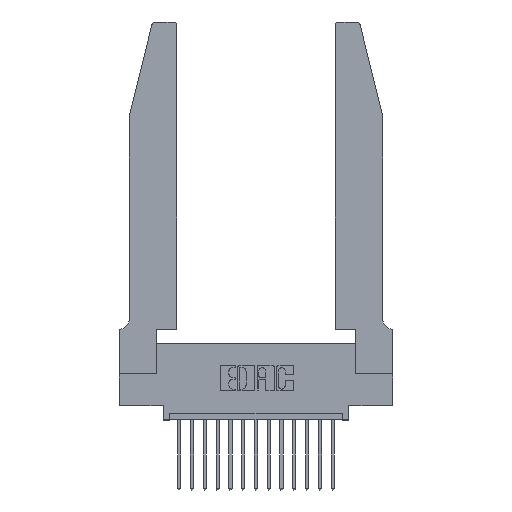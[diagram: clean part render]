
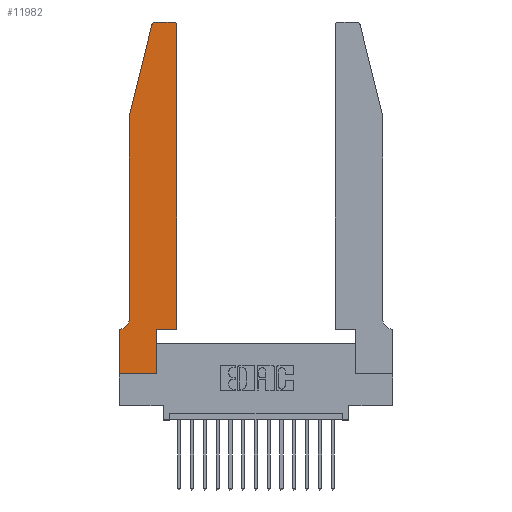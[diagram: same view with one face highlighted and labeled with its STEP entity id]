
A CAD part, top view. The second image highlights one B-rep face of the part: STEP entity #11982.
In plain terms, the highlighted planar face has unit normal (0, 0, 1).
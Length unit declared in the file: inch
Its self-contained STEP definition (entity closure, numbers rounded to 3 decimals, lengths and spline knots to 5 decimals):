
#133 = AXIS2_PLACEMENT_3D ( 'NONE', #11825, #15166, #6488 ) ;
#230 = EDGE_CURVE ( 'NONE', #1227, #12452, #915, .T. ) ;
#235 = CARTESIAN_POINT ( 'NONE',  ( 0., 0., 0.37 ) ) ;
#399 = CARTESIAN_POINT ( 'NONE',  ( 0.4505, 0.35, 0.37 ) ) ;
#492 = VERTEX_POINT ( 'NONE', #2204 ) ;
#555 = DIRECTION ( 'NONE',  ( -1., 0., 0. ) ) ;
#572 = CIRCLE ( 'NONE', #10017, 0.03 ) ;
#741 = LINE ( 'NONE', #235, #9506 ) ;
#759 = EDGE_CURVE ( 'NONE', #11024, #836, #6072, .T. ) ;
#790 = LINE ( 'NONE', #4311, #17644 ) ;
#828 = CARTESIAN_POINT ( 'NONE',  ( 0.0755, 2., 0.37 ) ) ;
#836 = VERTEX_POINT ( 'NONE', #18049 ) ;
#915 = LINE ( 'NONE', #828, #8326 ) ;
#1227 = VERTEX_POINT ( 'NONE', #9292 ) ;
#1251 = DIRECTION ( 'NONE',  ( 0., -1., 0. ) ) ;
#1268 = CIRCLE ( 'NONE', #8624, 0.07 ) ;
#1485 = EDGE_CURVE ( 'NONE', #11326, #2043, #12136, .T. ) ;
#1610 = ORIENTED_EDGE ( 'NONE', *, *, #5143, .T. ) ;
#1847 = CARTESIAN_POINT ( 'NONE',  ( 0.0755, 0.35, 0.37 ) ) ;
#1971 = EDGE_CURVE ( 'NONE', #2043, #492, #11453, .T. ) ;
#2043 = VERTEX_POINT ( 'NONE', #17514 ) ;
#2071 = ORIENTED_EDGE ( 'NONE', *, *, #759, .T. ) ;
#2204 = CARTESIAN_POINT ( 'NONE',  ( 0.4505, 0.35, 0.37 ) ) ;
#2301 = AXIS2_PLACEMENT_3D ( 'NONE', #8332, #8388, #2552 ) ;
#2552 = DIRECTION ( 'NONE',  ( 1., 0., 0. ) ) ;
#2676 = VECTOR ( 'NONE', #11862, 39.37008 ) ;
#3142 = CARTESIAN_POINT ( 'NONE',  ( 0.0755, 0.42, 0.37 ) ) ;
#3165 = DIRECTION ( 'NONE',  ( -1., 0., 0. ) ) ;
#3204 = CARTESIAN_POINT ( 'NONE',  ( 0., 0., 0.37 ) ) ;
#3379 = ORIENTED_EDGE ( 'NONE', *, *, #9868, .T. ) ;
#3469 = ORIENTED_EDGE ( 'NONE', *, *, #7093, .T. ) ;
#3857 = ORIENTED_EDGE ( 'NONE', *, *, #1971, .T. ) ;
#4170 = LINE ( 'NONE', #399, #8900 ) ;
#4178 = EDGE_CURVE ( 'NONE', #12461, #1227, #572, .T. ) ;
#4311 = CARTESIAN_POINT ( 'NONE',  ( 0.0755, 2., 0.37 ) ) ;
#4989 = DIRECTION ( 'NONE',  ( 0., 1., 0. ) ) ;
#5143 = EDGE_CURVE ( 'NONE', #12452, #11665, #790, .T. ) ;
#5204 = EDGE_CURVE ( 'NONE', #12669, #11326, #18302, .T. ) ;
#5235 = FACE_OUTER_BOUND ( 'NONE', #9716, .T. ) ;
#5941 = CARTESIAN_POINT ( 'NONE',  ( 0., 0., 0.37 ) ) ;
#6072 = CIRCLE ( 'NONE', #133, 0.03 ) ;
#6348 = ORIENTED_EDGE ( 'NONE', *, *, #230, .T. ) ;
#6377 = CARTESIAN_POINT ( 'NONE',  ( 0.0055, 0.35, 0.37 ) ) ;
#6461 = DIRECTION ( 'NONE',  ( -0.239, -0.971, 0. ) ) ;
#6488 = DIRECTION ( 'NONE',  ( 1., 0., 0. ) ) ;
#6499 = CARTESIAN_POINT ( 'NONE',  ( 0.284, 2.72, 0.37 ) ) ;
#6791 = CARTESIAN_POINT ( 'NONE',  ( 0.284, 2.75, 0.37 ) ) ;
#6950 = PLANE ( 'NONE',  #2301 ) ;
#7093 = EDGE_CURVE ( 'NONE', #492, #11024, #4170, .T. ) ;
#7434 = DIRECTION ( 'NONE',  ( 0., -1., 0. ) ) ;
#8117 = VERTEX_POINT ( 'NONE', #6377 ) ;
#8326 = VECTOR ( 'NONE', #6461, 39.37008 ) ;
#8332 = CARTESIAN_POINT ( 'NONE',  ( 0., 0.35, 0.37 ) ) ;
#8388 = DIRECTION ( 'NONE',  ( 0., 0., 1. ) ) ;
#8523 = VECTOR ( 'NONE', #4989, 39.37008 ) ;
#8624 = AXIS2_PLACEMENT_3D ( 'NONE', #13584, #9450, #16480 ) ;
#8760 = ORIENTED_EDGE ( 'NONE', *, *, #9781, .T. ) ;
#8900 = VECTOR ( 'NONE', #10963, 39.37008 ) ;
#9292 = CARTESIAN_POINT ( 'NONE',  ( 0.25487, 2.72718, 0.37 ) ) ;
#9450 = DIRECTION ( 'NONE',  ( 0., 0., -1. ) ) ;
#9506 = VECTOR ( 'NONE', #7434, 39.37008 ) ;
#9716 = EDGE_LOOP ( 'NONE', ( #15993, #14338, #6348, #1610, #3379, #8760, #15944, #17517, #10723, #3857, #3469, #2071 ) ) ;
#9781 = EDGE_CURVE ( 'NONE', #8117, #17095, #9831, .T. ) ;
#9831 = LINE ( 'NONE', #1847, #15447 ) ;
#9868 = EDGE_CURVE ( 'NONE', #11665, #8117, #1268, .T. ) ;
#10017 = AXIS2_PLACEMENT_3D ( 'NONE', #6499, #18011, #17128 ) ;
#10723 = ORIENTED_EDGE ( 'NONE', *, *, #1485, .T. ) ;
#10909 = CARTESIAN_POINT ( 'NONE',  ( 0.2865, 0.35, 0.37 ) ) ;
#10963 = DIRECTION ( 'NONE',  ( 0., 1., 0. ) ) ;
#11024 = VERTEX_POINT ( 'NONE', #14594 ) ;
#11326 = VERTEX_POINT ( 'NONE', #13890 ) ;
#11453 = LINE ( 'NONE', #14544, #2676 ) ;
#11665 = VERTEX_POINT ( 'NONE', #3142 ) ;
#11825 = CARTESIAN_POINT ( 'NONE',  ( 0.4205, 2.72, 0.37 ) ) ;
#11862 = DIRECTION ( 'NONE',  ( 1., 0., 0. ) ) ;
#11982 = ADVANCED_FACE ( 'NONE', ( #5235 ), #6950, .T. ) ;
#12136 = LINE ( 'NONE', #10909, #8523 ) ;
#12452 = VERTEX_POINT ( 'NONE', #18240 ) ;
#12461 = VERTEX_POINT ( 'NONE', #6791 ) ;
#12669 = VERTEX_POINT ( 'NONE', #3204 ) ;
#12739 = EDGE_CURVE ( 'NONE', #836, #12461, #14475, .T. ) ;
#13584 = CARTESIAN_POINT ( 'NONE',  ( 0.0055, 0.42, 0.37 ) ) ;
#13890 = CARTESIAN_POINT ( 'NONE',  ( 0.2865, 0., 0.37 ) ) ;
#14338 = ORIENTED_EDGE ( 'NONE', *, *, #4178, .T. ) ;
#14475 = LINE ( 'NONE', #17828, #14927 ) ;
#14484 = VECTOR ( 'NONE', #16036, 39.37008 ) ;
#14544 = CARTESIAN_POINT ( 'NONE',  ( 0.4505, 0.35, 0.37 ) ) ;
#14594 = CARTESIAN_POINT ( 'NONE',  ( 0.4505, 2.72, 0.37 ) ) ;
#14927 = VECTOR ( 'NONE', #555, 39.37008 ) ;
#15106 = CARTESIAN_POINT ( 'NONE',  ( 0., 0.35, 0.37 ) ) ;
#15166 = DIRECTION ( 'NONE',  ( 0., 0., 1. ) ) ;
#15447 = VECTOR ( 'NONE', #3165, 39.37008 ) ;
#15944 = ORIENTED_EDGE ( 'NONE', *, *, #17997, .T. ) ;
#15993 = ORIENTED_EDGE ( 'NONE', *, *, #12739, .T. ) ;
#16036 = DIRECTION ( 'NONE',  ( 1., 0., 0. ) ) ;
#16480 = DIRECTION ( 'NONE',  ( -1., 0., 0. ) ) ;
#17095 = VERTEX_POINT ( 'NONE', #15106 ) ;
#17128 = DIRECTION ( 'NONE',  ( 1., 0., 0. ) ) ;
#17514 = CARTESIAN_POINT ( 'NONE',  ( 0.2865, 0.35, 0.37 ) ) ;
#17517 = ORIENTED_EDGE ( 'NONE', *, *, #5204, .T. ) ;
#17644 = VECTOR ( 'NONE', #1251, 39.37008 ) ;
#17828 = CARTESIAN_POINT ( 'NONE',  ( 0.2605, 2.75, 0.37 ) ) ;
#17997 = EDGE_CURVE ( 'NONE', #17095, #12669, #741, .T. ) ;
#18011 = DIRECTION ( 'NONE',  ( 0., 0., 1. ) ) ;
#18049 = CARTESIAN_POINT ( 'NONE',  ( 0.4205, 2.75, 0.37 ) ) ;
#18240 = CARTESIAN_POINT ( 'NONE',  ( 0.0755, 2., 0.37 ) ) ;
#18302 = LINE ( 'NONE', #5941, #14484 ) ;
